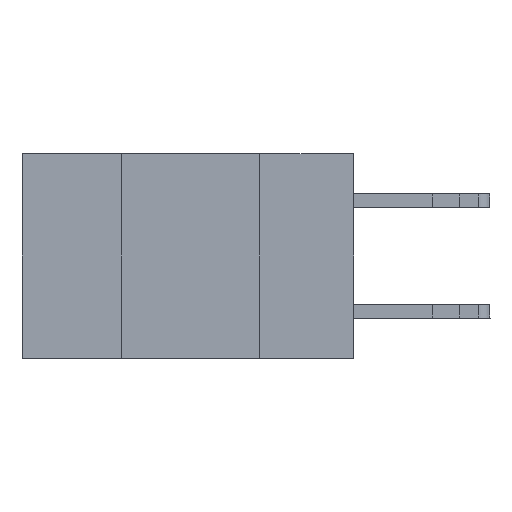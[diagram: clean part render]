
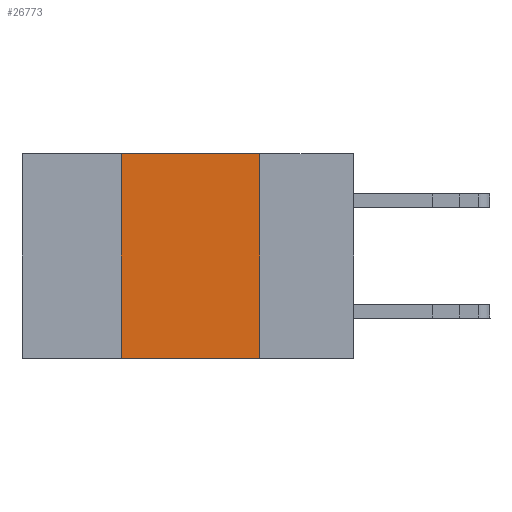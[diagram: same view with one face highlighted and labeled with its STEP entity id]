
A CAD part, left-side view. The second image highlights one B-rep face of the part: STEP entity #26773.
In plain terms, the highlighted planar face has unit normal (-1, 0, 0).
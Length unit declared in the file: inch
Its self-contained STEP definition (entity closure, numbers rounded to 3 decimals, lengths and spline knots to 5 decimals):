
#397 = CARTESIAN_POINT ( 'NONE',  ( 0., 0.17, -0.37 ) ) ;
#1639 = LINE ( 'NONE', #5181, #30621 ) ;
#2511 = DIRECTION ( 'NONE',  ( 0., -1., 0. ) ) ;
#3123 = CARTESIAN_POINT ( 'NONE',  ( 0., 0.42, 0. ) ) ;
#3154 = VERTEX_POINT ( 'NONE', #397 ) ;
#3464 = DIRECTION ( 'NONE',  ( 0., 0., -1. ) ) ;
#3917 = LINE ( 'NONE', #24836, #28191 ) ;
#4581 = DIRECTION ( 'NONE',  ( 0., -1., 0. ) ) ;
#4682 = FACE_OUTER_BOUND ( 'NONE', #29233, .T. ) ;
#5181 = CARTESIAN_POINT ( 'NONE',  ( 0., 0.6, -0.37 ) ) ;
#6203 = DIRECTION ( 'NONE',  ( 0., 0., -1. ) ) ;
#6292 = CARTESIAN_POINT ( 'NONE',  ( 0., 0.17, 0. ) ) ;
#7995 = VERTEX_POINT ( 'NONE', #6292 ) ;
#9154 = CARTESIAN_POINT ( 'NONE',  ( 0., 0.17, 0. ) ) ;
#9158 = AXIS2_PLACEMENT_3D ( 'NONE', #11191, #28923, #3464 ) ;
#10973 = PLANE ( 'NONE',  #9158 ) ;
#11067 = CARTESIAN_POINT ( 'NONE',  ( 0., 0.42, -0.37 ) ) ;
#11191 = CARTESIAN_POINT ( 'NONE',  ( 0., 0.6, 0. ) ) ;
#12315 = DIRECTION ( 'NONE',  ( 0., 0., 1. ) ) ;
#14194 = VECTOR ( 'NONE', #6203, 39.37008 ) ;
#16896 = VERTEX_POINT ( 'NONE', #11067 ) ;
#16914 = VECTOR ( 'NONE', #12315, 39.37008 ) ;
#18425 = EDGE_CURVE ( 'NONE', #16896, #23071, #30435, .T. ) ;
#21742 = LINE ( 'NONE', #9154, #14194 ) ;
#23071 = VERTEX_POINT ( 'NONE', #3123 ) ;
#23532 = ORIENTED_EDGE ( 'NONE', *, *, #23910, .F. ) ;
#23910 = EDGE_CURVE ( 'NONE', #7995, #3154, #21742, .T. ) ;
#24190 = ORIENTED_EDGE ( 'NONE', *, *, #18425, .F. ) ;
#24836 = CARTESIAN_POINT ( 'NONE',  ( 0., 0.6, 0. ) ) ;
#26400 = EDGE_CURVE ( 'NONE', #23071, #7995, #3917, .T. ) ;
#26773 = ADVANCED_FACE ( 'NONE', ( #4682 ), #10973, .F. ) ;
#27500 = CARTESIAN_POINT ( 'NONE',  ( 0., 0.42, 0. ) ) ;
#28191 = VECTOR ( 'NONE', #4581, 39.37008 ) ;
#28759 = ORIENTED_EDGE ( 'NONE', *, *, #31739, .T. ) ;
#28923 = DIRECTION ( 'NONE',  ( 1., 0., 0. ) ) ;
#29214 = ORIENTED_EDGE ( 'NONE', *, *, #26400, .F. ) ;
#29233 = EDGE_LOOP ( 'NONE', ( #23532, #29214, #24190, #28759 ) ) ;
#30435 = LINE ( 'NONE', #27500, #16914 ) ;
#30621 = VECTOR ( 'NONE', #2511, 39.37008 ) ;
#31739 = EDGE_CURVE ( 'NONE', #16896, #3154, #1639, .T. ) ;
